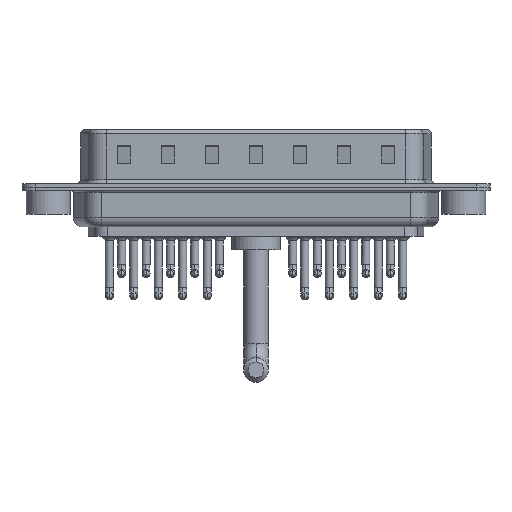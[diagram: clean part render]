
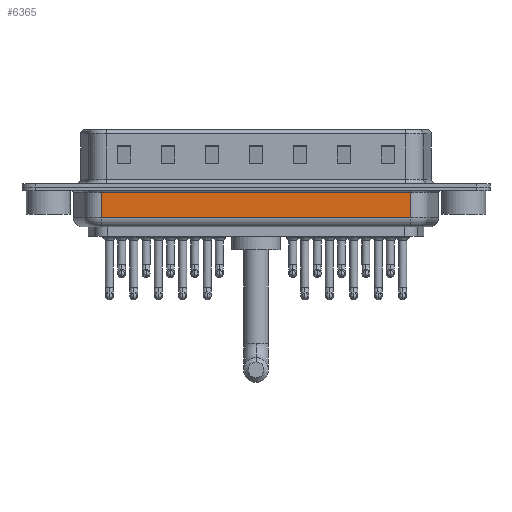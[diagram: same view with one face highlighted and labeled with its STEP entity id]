
A CAD part, front view. The second image highlights one B-rep face of the part: STEP entity #6365.
In plain terms, the highlighted planar face has unit normal (0, -1, 0).
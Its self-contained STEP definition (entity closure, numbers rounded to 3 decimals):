
#705 = VERTEX_POINT ( 'NONE', #23971 ) ;
#1831 = CARTESIAN_POINT ( 'NONE',  ( 6.006, -5.35, -3.5 ) ) ;
#3752 = ORIENTED_EDGE ( 'NONE', *, *, #14965, .T. ) ;
#4761 = EDGE_CURVE ( 'NONE', #21506, #705, #13977, .T. ) ;
#5020 = ORIENTED_EDGE ( 'NONE', *, *, #4761, .T. ) ;
#5029 = DIRECTION ( 'NONE',  ( 1., 0., 0. ) ) ;
#5539 = DIRECTION ( 'NONE',  ( 0., 0., 1. ) ) ;
#6365 = ADVANCED_FACE ( 'NONE', ( #9367 ), #7651, .F. ) ;
#6931 = CARTESIAN_POINT ( 'NONE',  ( 6.006, -5.35, -0.65 ) ) ;
#7036 = LINE ( 'NONE', #22399, #12306 ) ;
#7110 = VERTEX_POINT ( 'NONE', #6931 ) ;
#7651 = PLANE ( 'NONE',  #15367 ) ;
#8062 = CARTESIAN_POINT ( 'NONE',  ( 41.044, -5.35, -4.5 ) ) ;
#9367 = FACE_OUTER_BOUND ( 'NONE', #25399, .T. ) ;
#12306 = VECTOR ( 'NONE', #23565, 1000. ) ;
#12879 = VERTEX_POINT ( 'NONE', #1831 ) ;
#13977 = LINE ( 'NONE', #8062, #20332 ) ;
#14366 = DIRECTION ( 'NONE',  ( 0., 0., 1. ) ) ;
#14965 = EDGE_CURVE ( 'NONE', #705, #7110, #7036, .T. ) ;
#15033 = LINE ( 'NONE', #23010, #23708 ) ;
#15367 = AXIS2_PLACEMENT_3D ( 'NONE', #23520, #17633, #5539 ) ;
#16179 = LINE ( 'NONE', #16566, #18398 ) ;
#16566 = CARTESIAN_POINT ( 'NONE',  ( 6.006, -5.35, -4.5 ) ) ;
#17633 = DIRECTION ( 'NONE',  ( 0., 1., 0. ) ) ;
#18398 = VECTOR ( 'NONE', #24148, 1000. ) ;
#19287 = EDGE_CURVE ( 'NONE', #12879, #7110, #16179, .T. ) ;
#20332 = VECTOR ( 'NONE', #14366, 1000. ) ;
#20375 = EDGE_CURVE ( 'NONE', #12879, #21506, #15033, .T. ) ;
#21506 = VERTEX_POINT ( 'NONE', #22377 ) ;
#22377 = CARTESIAN_POINT ( 'NONE',  ( 41.044, -5.35, -3.5 ) ) ;
#22399 = CARTESIAN_POINT ( 'NONE',  ( 6.006, -5.35, -0.65 ) ) ;
#23010 = CARTESIAN_POINT ( 'NONE',  ( 6.006, -5.35, -3.5 ) ) ;
#23520 = CARTESIAN_POINT ( 'NONE',  ( 6.006, -5.35, -4.5 ) ) ;
#23565 = DIRECTION ( 'NONE',  ( -1., 0., 0. ) ) ;
#23708 = VECTOR ( 'NONE', #5029, 1000. ) ;
#23971 = CARTESIAN_POINT ( 'NONE',  ( 41.044, -5.35, -0.65 ) ) ;
#24148 = DIRECTION ( 'NONE',  ( 0., 0., 1. ) ) ;
#25110 = ORIENTED_EDGE ( 'NONE', *, *, #19287, .F. ) ;
#25154 = ORIENTED_EDGE ( 'NONE', *, *, #20375, .T. ) ;
#25399 = EDGE_LOOP ( 'NONE', ( #25110, #25154, #5020, #3752 ) ) ;
